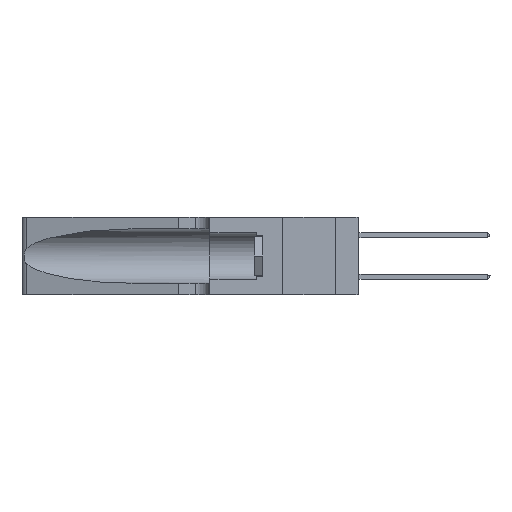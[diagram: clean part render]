
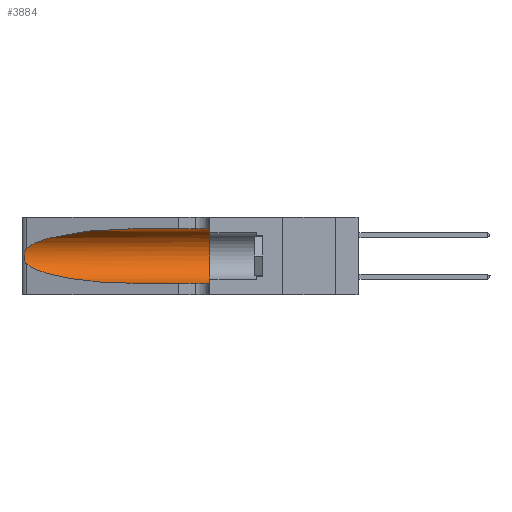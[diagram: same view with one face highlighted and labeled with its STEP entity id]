
A CAD part, left-side view. The second image highlights one B-rep face of the part: STEP entity #3884.
In plain terms, the highlighted cylindrical face has radius 3.308 mm (diameter 6.617 mm), a partial arc.
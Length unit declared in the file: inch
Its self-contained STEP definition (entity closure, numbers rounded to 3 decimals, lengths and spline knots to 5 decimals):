
#120 = ORIENTED_EDGE ( 'NONE', *, *, #2918, .T. ) ;
#144 = CARTESIAN_POINT ( 'NONE',  ( 0.25487, 1.22718, 0.22369 ) ) ;
#253 = EDGE_CURVE ( 'NONE', #22665, #14067, #1621, .T. ) ;
#1358 = CARTESIAN_POINT ( 'NONE',  ( 0.25787, 1.23484, 0.2124 ) ) ;
#1520 = AXIS2_PLACEMENT_3D ( 'NONE', #27766, #28559, #21678 ) ;
#1621 = CIRCLE ( 'NONE', #15016, 0.13025 ) ;
#1952 = EDGE_CURVE ( 'NONE', #7578, #19504, #28441, .T. ) ;
#2258 = CARTESIAN_POINT ( 'NONE',  ( 0.1305, 0.72297, 0.31525 ) ) ;
#2803 = CARTESIAN_POINT ( 'NONE',  ( 0.26018, 1.23835, 0.19895 ) ) ;
#2918 = EDGE_CURVE ( 'NONE', #19504, #4756, #29386, .T. ) ;
#3326 = CARTESIAN_POINT ( 'NONE',  ( 0.25639, 1.23186, 0.15144 ) ) ;
#3884 = ADVANCED_FACE ( 'NONE', ( #17314 ), #12543, .F. ) ;
#3928 = CARTESIAN_POINT ( 'NONE',  ( 0.1305, 0.72297, 0.31525 ) ) ;
#4229 = CARTESIAN_POINT ( 'NONE',  ( 0.1305, 0.35, 0.05475 ) ) ;
#4756 = VERTEX_POINT ( 'NONE', #8552 ) ;
#5452 = ORIENTED_EDGE ( 'NONE', *, *, #19672, .F. ) ;
#5945 = CARTESIAN_POINT ( 'NONE',  ( 0.2373, 1.15595, 0.08982 ) ) ;
#6822 = CARTESIAN_POINT ( 'NONE',  ( 0.26075, 1.23896, 0.19203 ) ) ;
#7578 = VERTEX_POINT ( 'NONE', #3928 ) ;
#7684 = DIRECTION ( 'NONE',  ( 0., 1., 0. ) ) ;
#8117 = CARTESIAN_POINT ( 'NONE',  ( 0.1305, 1.61858, 0.31525 ) ) ;
#8429 = CARTESIAN_POINT ( 'NONE',  ( 0.25487, 1.22718, 0.14631 ) ) ;
#8552 = CARTESIAN_POINT ( 'NONE',  ( 0.25487, 1.22718, 0.14631 ) ) ;
#9489 = CARTESIAN_POINT ( 'NONE',  ( 0.25555, 1.22994, 0.2215 ) ) ;
#10398 = EDGE_CURVE ( 'NONE', #4756, #16748, #11950, .T. ) ;
#10671 = VECTOR ( 'NONE', #23994, 39.37008 ) ;
#10829 = DIRECTION ( 'NONE',  ( 0., -1., 0. ) ) ;
#11950 =( BOUNDED_CURVE ( )  B_SPLINE_CURVE ( 3, ( #27159, #5945, #22506, #25011 ),
 .UNSPECIFIED., .F., .F. ) 
 B_SPLINE_CURVE_WITH_KNOTS ( ( 4, 4 ),
 ( 3.44316, 4.71239 ),
 .UNSPECIFIED. ) 
 CURVE ( )  GEOMETRIC_REPRESENTATION_ITEM ( )  RATIONAL_B_SPLINE_CURVE ( ( 1., 0.87, 0.87, 1. ) ) 
 REPRESENTATION_ITEM ( '' )  );
#12449 = CARTESIAN_POINT ( 'NONE',  ( 0.1305, 1.61858, 0.05475 ) ) ;
#12543 = CYLINDRICAL_SURFACE ( 'NONE', #1520, 0.13025 ) ;
#12549 = CARTESIAN_POINT ( 'NONE',  ( 0.25639, 1.23184, 0.21858 ) ) ;
#12780 = CARTESIAN_POINT ( 'NONE',  ( 0.1305, 0.35, 0.185 ) ) ;
#13910 = EDGE_LOOP ( 'NONE', ( #14858, #120, #26485, #29833, #26084, #5452 ) ) ;
#14067 = VERTEX_POINT ( 'NONE', #4229 ) ;
#14118 = CARTESIAN_POINT ( 'NONE',  ( 0.25487, 1.22718, 0.22369 ) ) ;
#14245 = CARTESIAN_POINT ( 'NONE',  ( 0.18966, 0.96281, 0.31525 ) ) ;
#14858 = ORIENTED_EDGE ( 'NONE', *, *, #1952, .T. ) ;
#15016 = AXIS2_PLACEMENT_3D ( 'NONE', #12780, #7684, #17602 ) ;
#15195 = CARTESIAN_POINT ( 'NONE',  ( 0.25789, 1.23486, 0.15765 ) ) ;
#16748 = VERTEX_POINT ( 'NONE', #16881 ) ;
#16881 = CARTESIAN_POINT ( 'NONE',  ( 0.1305, 0.72297, 0.05475 ) ) ;
#17314 = FACE_OUTER_BOUND ( 'NONE', #13910, .T. ) ;
#17602 = DIRECTION ( 'NONE',  ( 0., 0., 1. ) ) ;
#18877 = CARTESIAN_POINT ( 'NONE',  ( 0.2373, 1.15595, 0.28018 ) ) ;
#19504 = VERTEX_POINT ( 'NONE', #28728 ) ;
#19672 = EDGE_CURVE ( 'NONE', #7578, #22665, #27141, .T. ) ;
#21678 = DIRECTION ( 'NONE',  ( 0., 0., -1. ) ) ;
#22343 = EDGE_CURVE ( 'NONE', #16748, #14067, #29968, .T. ) ;
#22506 = CARTESIAN_POINT ( 'NONE',  ( 0.18966, 0.96281, 0.05475 ) ) ;
#22665 = VERTEX_POINT ( 'NONE', #30099 ) ;
#23582 = CARTESIAN_POINT ( 'NONE',  ( 0.26075, 1.23896, 0.178 ) ) ;
#23679 = CARTESIAN_POINT ( 'NONE',  ( 0.26017, 1.23833, 0.17102 ) ) ;
#23994 = DIRECTION ( 'NONE',  ( 0., -1., 0. ) ) ;
#25011 = CARTESIAN_POINT ( 'NONE',  ( 0.1305, 0.72297, 0.05475 ) ) ;
#26067 = CARTESIAN_POINT ( 'NONE',  ( 0.25856, 1.23593, 0.16098 ) ) ;
#26084 = ORIENTED_EDGE ( 'NONE', *, *, #253, .F. ) ;
#26485 = ORIENTED_EDGE ( 'NONE', *, *, #10398, .T. ) ;
#27141 = LINE ( 'NONE', #8117, #27896 ) ;
#27159 = CARTESIAN_POINT ( 'NONE',  ( 0.25487, 1.22718, 0.14631 ) ) ;
#27766 = CARTESIAN_POINT ( 'NONE',  ( 0.1305, 1.61858, 0.185 ) ) ;
#27896 = VECTOR ( 'NONE', #10829, 39.37008 ) ;
#28328 = CARTESIAN_POINT ( 'NONE',  ( 0.25854, 1.2359, 0.20912 ) ) ;
#28441 =( BOUNDED_CURVE ( )  B_SPLINE_CURVE ( 3, ( #2258, #14245, #18877, #144 ),
 .UNSPECIFIED., .F., .F. ) 
 B_SPLINE_CURVE_WITH_KNOTS ( ( 4, 4 ),
 ( 1.5708, 2.84003 ),
 .UNSPECIFIED. ) 
 CURVE ( )  GEOMETRIC_REPRESENTATION_ITEM ( )  RATIONAL_B_SPLINE_CURVE ( ( 1., 0.87, 0.87, 1. ) ) 
 REPRESENTATION_ITEM ( '' )  );
#28559 = DIRECTION ( 'NONE',  ( 0., -1., 0. ) ) ;
#28728 = CARTESIAN_POINT ( 'NONE',  ( 0.25487, 1.22718, 0.22369 ) ) ;
#29386 = B_SPLINE_CURVE_WITH_KNOTS ( 'NONE', 3,
 ( #14118, #9489, #12549, #1358, #28328, #2803, #6822, #23582, #23679, #26067, #15195, #3326, #29992, #8429 ),
 .UNSPECIFIED., .F., .F.,
 ( 4, 2, 2, 2, 2, 2, 4 ),
 ( 0., 0.00027, 0.00053, 0.00107, 0.0016, 0.00187, 0.00214 ),
 .UNSPECIFIED. ) ;
#29833 = ORIENTED_EDGE ( 'NONE', *, *, #22343, .T. ) ;
#29968 = LINE ( 'NONE', #12449, #10671 ) ;
#29992 = CARTESIAN_POINT ( 'NONE',  ( 0.25555, 1.22993, 0.14849 ) ) ;
#30099 = CARTESIAN_POINT ( 'NONE',  ( 0.1305, 0.35, 0.31525 ) ) ;
